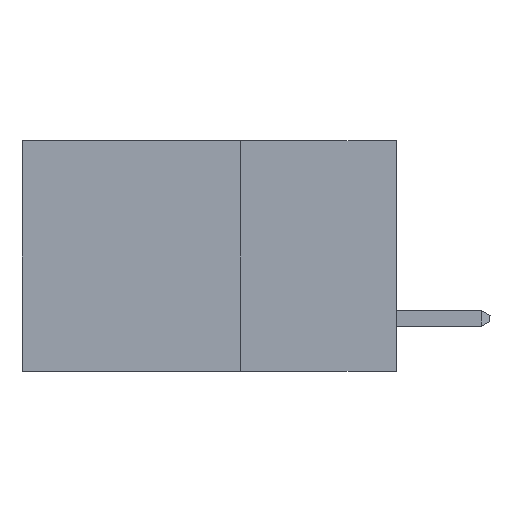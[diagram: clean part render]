
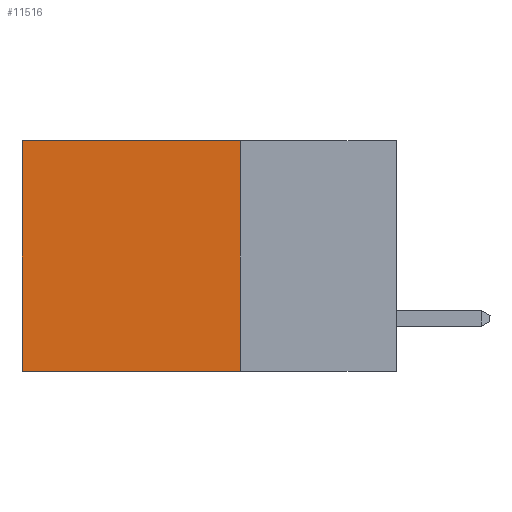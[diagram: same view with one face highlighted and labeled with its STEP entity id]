
A CAD part, left-side view. The second image highlights one B-rep face of the part: STEP entity #11516.
In plain terms, the highlighted planar face has unit normal (-1, 0, 0).
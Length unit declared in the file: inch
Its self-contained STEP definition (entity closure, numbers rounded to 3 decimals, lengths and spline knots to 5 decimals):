
#24 = VERTEX_POINT ( 'NONE', #4559 ) ;
#1171 = FACE_OUTER_BOUND ( 'NONE', #11779, .T. ) ;
#1285 = EDGE_CURVE ( 'NONE', #24, #12431, #13951, .T. ) ;
#1363 = CARTESIAN_POINT ( 'NONE',  ( 0.2615, 0.25, -0.37 ) ) ;
#1450 = VECTOR ( 'NONE', #7556, 39.37008 ) ;
#1815 = VECTOR ( 'NONE', #10626, 39.37008 ) ;
#3137 = CARTESIAN_POINT ( 'NONE',  ( 0.2615, 0.25, -0.37 ) ) ;
#4148 = PLANE ( 'NONE',  #8515 ) ;
#4558 = ORIENTED_EDGE ( 'NONE', *, *, #7481, .T. ) ;
#4559 = CARTESIAN_POINT ( 'NONE',  ( 0.2615, 0.6, 0. ) ) ;
#4606 = LINE ( 'NONE', #9973, #1450 ) ;
#4893 = ORIENTED_EDGE ( 'NONE', *, *, #12658, .F. ) ;
#5386 = CARTESIAN_POINT ( 'NONE',  ( 0.2615, 0.25, -0.37 ) ) ;
#6013 = VECTOR ( 'NONE', #11585, 39.37008 ) ;
#6581 = DIRECTION ( 'NONE',  ( 1., 0., 0. ) ) ;
#6661 = VERTEX_POINT ( 'NONE', #1363 ) ;
#7251 = DIRECTION ( 'NONE',  ( 0., 0., -1. ) ) ;
#7481 = EDGE_CURVE ( 'NONE', #9969, #24, #7834, .T. ) ;
#7556 = DIRECTION ( 'NONE',  ( 0., 0., -1. ) ) ;
#7834 = LINE ( 'NONE', #10684, #1815 ) ;
#8136 = ORIENTED_EDGE ( 'NONE', *, *, #1285, .T. ) ;
#8338 = CARTESIAN_POINT ( 'NONE',  ( 0.2615, 0.6, -0.37 ) ) ;
#8515 = AXIS2_PLACEMENT_3D ( 'NONE', #5386, #6581, #14704 ) ;
#9268 = CARTESIAN_POINT ( 'NONE',  ( 0.2615, 0.6, -0.37 ) ) ;
#9969 = VERTEX_POINT ( 'NONE', #11808 ) ;
#9973 = CARTESIAN_POINT ( 'NONE',  ( 0.2615, 0.25, -0.37 ) ) ;
#10131 = ORIENTED_EDGE ( 'NONE', *, *, #11594, .F. ) ;
#10626 = DIRECTION ( 'NONE',  ( 0., 1., 0. ) ) ;
#10684 = CARTESIAN_POINT ( 'NONE',  ( 0.2615, 0.25, 0. ) ) ;
#10992 = VECTOR ( 'NONE', #7251, 39.37008 ) ;
#11516 = ADVANCED_FACE ( 'NONE', ( #1171 ), #4148, .F. ) ;
#11585 = DIRECTION ( 'NONE',  ( 0., 1., 0. ) ) ;
#11594 = EDGE_CURVE ( 'NONE', #6661, #12431, #14898, .T. ) ;
#11779 = EDGE_LOOP ( 'NONE', ( #8136, #10131, #4893, #4558 ) ) ;
#11808 = CARTESIAN_POINT ( 'NONE',  ( 0.2615, 0.25, 0. ) ) ;
#12431 = VERTEX_POINT ( 'NONE', #8338 ) ;
#12658 = EDGE_CURVE ( 'NONE', #9969, #6661, #4606, .T. ) ;
#13951 = LINE ( 'NONE', #9268, #10992 ) ;
#14704 = DIRECTION ( 'NONE',  ( 0., 0., -1. ) ) ;
#14898 = LINE ( 'NONE', #3137, #6013 ) ;
